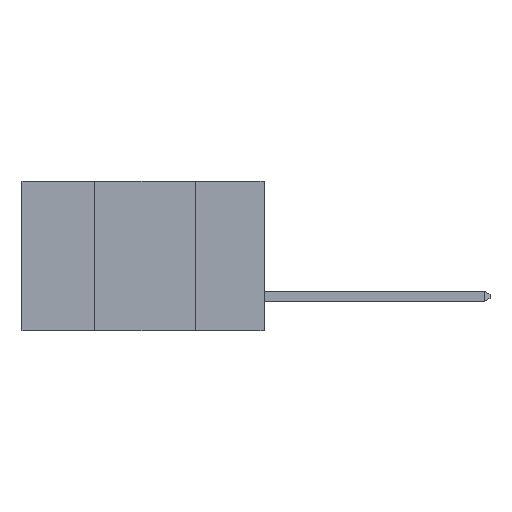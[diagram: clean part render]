
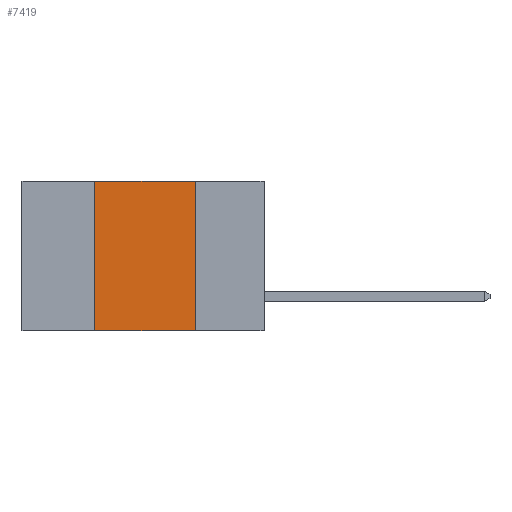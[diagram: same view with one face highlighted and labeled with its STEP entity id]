
A CAD part, left-side view. The second image highlights one B-rep face of the part: STEP entity #7419.
In plain terms, the highlighted planar face has unit normal (-1, 0, 0).
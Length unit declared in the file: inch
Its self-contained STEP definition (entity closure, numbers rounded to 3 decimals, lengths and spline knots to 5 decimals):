
#23 = DIRECTION ( 'NONE',  ( 1., 0., 0. ) ) ;
#110 = ORIENTED_EDGE ( 'NONE', *, *, #1021, .T. ) ;
#127 = EDGE_CURVE ( 'NONE', #3535, #7032, #4895, .T. ) ;
#496 = VERTEX_POINT ( 'NONE', #6669 ) ;
#1021 = EDGE_CURVE ( 'NONE', #3933, #496, #1318, .T. ) ;
#1257 = PLANE ( 'NONE',  #7451 ) ;
#1318 = LINE ( 'NONE', #3834, #10411 ) ;
#1675 = LINE ( 'NONE', #1892, #10999 ) ;
#1892 = CARTESIAN_POINT ( 'NONE',  ( 0., 0.17, -0.37 ) ) ;
#2214 = ORIENTED_EDGE ( 'NONE', *, *, #127, .F. ) ;
#2590 = CARTESIAN_POINT ( 'NONE',  ( 0., 0.42, 0. ) ) ;
#2647 = VECTOR ( 'NONE', #2978, 39.37008 ) ;
#2706 = CARTESIAN_POINT ( 'NONE',  ( 0., 0.6, 0. ) ) ;
#2978 = DIRECTION ( 'NONE',  ( 0., -1., 0. ) ) ;
#3535 = VERTEX_POINT ( 'NONE', #2590 ) ;
#3834 = CARTESIAN_POINT ( 'NONE',  ( 0., 0.6, -0.37 ) ) ;
#3933 = VERTEX_POINT ( 'NONE', #4211 ) ;
#4211 = CARTESIAN_POINT ( 'NONE',  ( 0., 0.42, -0.37 ) ) ;
#4485 = ORIENTED_EDGE ( 'NONE', *, *, #7127, .F. ) ;
#4895 = LINE ( 'NONE', #2706, #2647 ) ;
#5113 = CARTESIAN_POINT ( 'NONE',  ( 0., 0.6, 0. ) ) ;
#5172 = DIRECTION ( 'NONE',  ( 0., -1., 0. ) ) ;
#5337 = DIRECTION ( 'NONE',  ( 0., 0., -1. ) ) ;
#5971 = LINE ( 'NONE', #8641, #8400 ) ;
#6669 = CARTESIAN_POINT ( 'NONE',  ( 0., 0.17, -0.37 ) ) ;
#7032 = VERTEX_POINT ( 'NONE', #10926 ) ;
#7127 = EDGE_CURVE ( 'NONE', #3933, #3535, #5971, .T. ) ;
#7419 = ADVANCED_FACE ( 'NONE', ( #10886 ), #1257, .F. ) ;
#7451 = AXIS2_PLACEMENT_3D ( 'NONE', #5113, #23, #11328 ) ;
#8400 = VECTOR ( 'NONE', #8573, 39.37008 ) ;
#8573 = DIRECTION ( 'NONE',  ( 0., 0., 1. ) ) ;
#8641 = CARTESIAN_POINT ( 'NONE',  ( 0., 0.42, -0.37 ) ) ;
#8996 = ORIENTED_EDGE ( 'NONE', *, *, #9172, .F. ) ;
#9172 = EDGE_CURVE ( 'NONE', #7032, #496, #1675, .T. ) ;
#9551 = EDGE_LOOP ( 'NONE', ( #8996, #2214, #4485, #110 ) ) ;
#10411 = VECTOR ( 'NONE', #5172, 39.37008 ) ;
#10886 = FACE_OUTER_BOUND ( 'NONE', #9551, .T. ) ;
#10926 = CARTESIAN_POINT ( 'NONE',  ( 0., 0.17, 0. ) ) ;
#10999 = VECTOR ( 'NONE', #5337, 39.37008 ) ;
#11328 = DIRECTION ( 'NONE',  ( 0., 0., -1. ) ) ;
